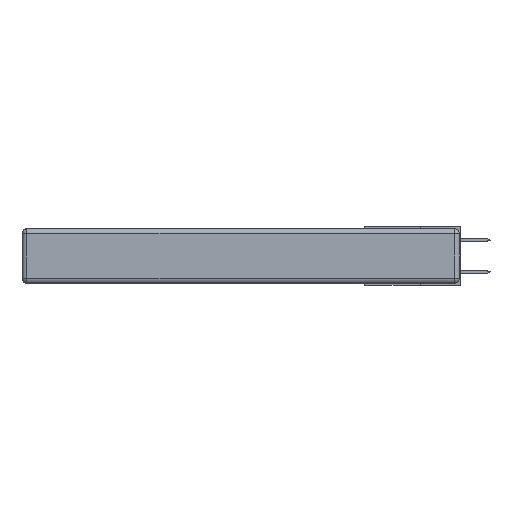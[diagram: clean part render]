
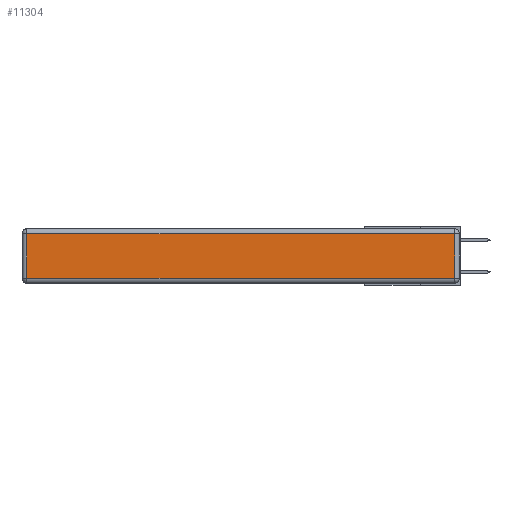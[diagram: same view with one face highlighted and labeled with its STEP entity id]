
A CAD part, left-side view. The second image highlights one B-rep face of the part: STEP entity #11304.
In plain terms, the highlighted planar face has unit normal (-1, 0, 0).
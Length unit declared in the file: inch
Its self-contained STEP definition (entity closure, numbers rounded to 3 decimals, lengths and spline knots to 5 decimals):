
#891 = VECTOR ( 'NONE', #19375, 39.37008 ) ;
#1331 = PLANE ( 'NONE',  #14035 ) ;
#2207 = CARTESIAN_POINT ( 'NONE',  ( 0., 2.72, -0.03 ) ) ;
#2490 = EDGE_CURVE ( 'NONE', #9971, #17792, #4724, .T. ) ;
#4724 = LINE ( 'NONE', #12590, #891 ) ;
#4960 = ORIENTED_EDGE ( 'NONE', *, *, #14937, .T. ) ;
#5093 = CARTESIAN_POINT ( 'NONE',  ( 0., 0.03, -0.313 ) ) ;
#6037 = DIRECTION ( 'NONE',  ( 0., 0., -1. ) ) ;
#6384 = EDGE_CURVE ( 'NONE', #15124, #9971, #12413, .T. ) ;
#9971 = VERTEX_POINT ( 'NONE', #10090 ) ;
#10090 = CARTESIAN_POINT ( 'NONE',  ( 0., 2.72, -0.313 ) ) ;
#10325 = CARTESIAN_POINT ( 'NONE',  ( 0., 0.03, -0.03 ) ) ;
#10883 = ORIENTED_EDGE ( 'NONE', *, *, #2490, .T. ) ;
#11304 = ADVANCED_FACE ( 'NONE', ( #24918 ), #1331, .T. ) ;
#12413 = LINE ( 'NONE', #17250, #17326 ) ;
#12590 = CARTESIAN_POINT ( 'NONE',  ( 0., 0., -0.313 ) ) ;
#14035 = AXIS2_PLACEMENT_3D ( 'NONE', #17110, #23938, #15509 ) ;
#14937 = EDGE_CURVE ( 'NONE', #17792, #26232, #26694, .T. ) ;
#15124 = VERTEX_POINT ( 'NONE', #2207 ) ;
#15509 = DIRECTION ( 'NONE',  ( 0., 0., 1. ) ) ;
#17110 = CARTESIAN_POINT ( 'NONE',  ( 0., 0., -0.343 ) ) ;
#17250 = CARTESIAN_POINT ( 'NONE',  ( 0., 2.72, -0.343 ) ) ;
#17255 = DIRECTION ( 'NONE',  ( 0., 0., 1. ) ) ;
#17326 = VECTOR ( 'NONE', #6037, 39.37008 ) ;
#17469 = VECTOR ( 'NONE', #24603, 39.37008 ) ;
#17792 = VERTEX_POINT ( 'NONE', #5093 ) ;
#18125 = CARTESIAN_POINT ( 'NONE',  ( 0., 2.75, -0.03 ) ) ;
#19183 = ORIENTED_EDGE ( 'NONE', *, *, #27104, .T. ) ;
#19375 = DIRECTION ( 'NONE',  ( 0., -1., 0. ) ) ;
#23394 = LINE ( 'NONE', #18125, #17469 ) ;
#23858 = VECTOR ( 'NONE', #17255, 39.37008 ) ;
#23878 = CARTESIAN_POINT ( 'NONE',  ( 0., 0.03, -0.343 ) ) ;
#23938 = DIRECTION ( 'NONE',  ( -1., 0., 0. ) ) ;
#24323 = ORIENTED_EDGE ( 'NONE', *, *, #6384, .T. ) ;
#24603 = DIRECTION ( 'NONE',  ( 0., 1., 0. ) ) ;
#24617 = EDGE_LOOP ( 'NONE', ( #10883, #4960, #19183, #24323 ) ) ;
#24918 = FACE_OUTER_BOUND ( 'NONE', #24617, .T. ) ;
#26232 = VERTEX_POINT ( 'NONE', #10325 ) ;
#26694 = LINE ( 'NONE', #23878, #23858 ) ;
#27104 = EDGE_CURVE ( 'NONE', #26232, #15124, #23394, .T. ) ;
